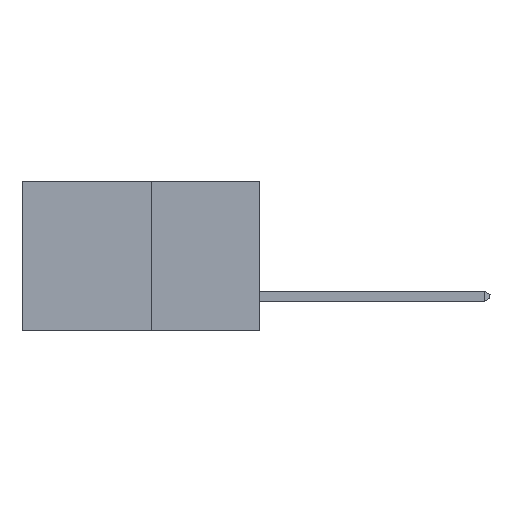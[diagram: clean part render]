
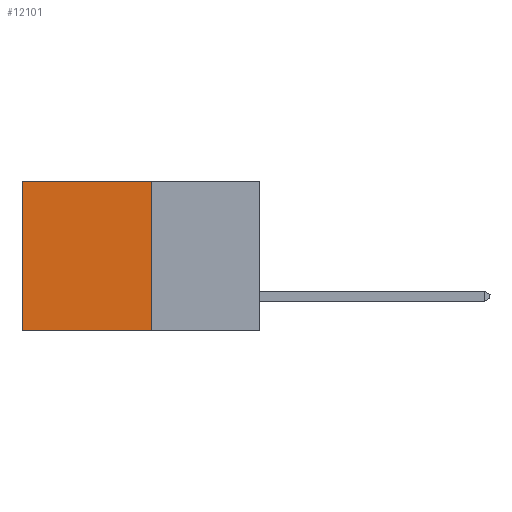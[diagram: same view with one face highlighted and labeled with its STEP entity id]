
A CAD part, left-side view. The second image highlights one B-rep face of the part: STEP entity #12101.
In plain terms, the highlighted planar face has unit normal (-1, 0, 0).
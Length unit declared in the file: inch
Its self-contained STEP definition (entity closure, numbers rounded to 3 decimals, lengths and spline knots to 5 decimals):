
#25 = EDGE_CURVE ( 'NONE', #5325, #9917, #3772, .T. ) ;
#230 = DIRECTION ( 'NONE',  ( 0., 1., 0. ) ) ;
#1642 = DIRECTION ( 'NONE',  ( 0., 0., -1. ) ) ;
#2413 = CARTESIAN_POINT ( 'NONE',  ( 0.277, 0.27, -0.37 ) ) ;
#2715 = VERTEX_POINT ( 'NONE', #15488 ) ;
#3116 = CARTESIAN_POINT ( 'NONE',  ( 0.277, 0.27, 0. ) ) ;
#3772 = LINE ( 'NONE', #2413, #10644 ) ;
#3780 = FACE_OUTER_BOUND ( 'NONE', #9572, .T. ) ;
#4789 = VECTOR ( 'NONE', #6156, 39.37008 ) ;
#4845 = ORIENTED_EDGE ( 'NONE', *, *, #15088, .F. ) ;
#5325 = VERTEX_POINT ( 'NONE', #3116 ) ;
#5935 = DIRECTION ( 'NONE',  ( 1., 0., 0. ) ) ;
#6156 = DIRECTION ( 'NONE',  ( 0., 1., 0. ) ) ;
#6356 = VERTEX_POINT ( 'NONE', #16155 ) ;
#6794 = CARTESIAN_POINT ( 'NONE',  ( 0.277, 0.27, -0.37 ) ) ;
#7668 = ORIENTED_EDGE ( 'NONE', *, *, #9513, .T. ) ;
#8619 = VECTOR ( 'NONE', #230, 39.37008 ) ;
#8708 = ORIENTED_EDGE ( 'NONE', *, *, #25, .F. ) ;
#8945 = VECTOR ( 'NONE', #12753, 39.37008 ) ;
#9238 = LINE ( 'NONE', #10202, #4789 ) ;
#9513 = EDGE_CURVE ( 'NONE', #5325, #6356, #15731, .T. ) ;
#9572 = EDGE_LOOP ( 'NONE', ( #10305, #4845, #8708, #7668 ) ) ;
#9917 = VERTEX_POINT ( 'NONE', #6794 ) ;
#9934 = CARTESIAN_POINT ( 'NONE',  ( 0.277, 0.27, -0.37 ) ) ;
#10202 = CARTESIAN_POINT ( 'NONE',  ( 0.277, 0.27, -0.37 ) ) ;
#10305 = ORIENTED_EDGE ( 'NONE', *, *, #12206, .T. ) ;
#10644 = VECTOR ( 'NONE', #1642, 39.37008 ) ;
#12101 = ADVANCED_FACE ( 'NONE', ( #3780 ), #12588, .F. ) ;
#12206 = EDGE_CURVE ( 'NONE', #6356, #2715, #12898, .T. ) ;
#12588 = PLANE ( 'NONE',  #14224 ) ;
#12753 = DIRECTION ( 'NONE',  ( 0., 0., -1. ) ) ;
#12898 = LINE ( 'NONE', #15532, #8945 ) ;
#14048 = CARTESIAN_POINT ( 'NONE',  ( 0.277, 0.27, 0. ) ) ;
#14224 = AXIS2_PLACEMENT_3D ( 'NONE', #9934, #5935, #15302 ) ;
#15088 = EDGE_CURVE ( 'NONE', #9917, #2715, #9238, .T. ) ;
#15302 = DIRECTION ( 'NONE',  ( 0., 0., -1. ) ) ;
#15488 = CARTESIAN_POINT ( 'NONE',  ( 0.277, 0.59, -0.37 ) ) ;
#15532 = CARTESIAN_POINT ( 'NONE',  ( 0.277, 0.59, -0.37 ) ) ;
#15731 = LINE ( 'NONE', #14048, #8619 ) ;
#16155 = CARTESIAN_POINT ( 'NONE',  ( 0.277, 0.59, 0. ) ) ;
